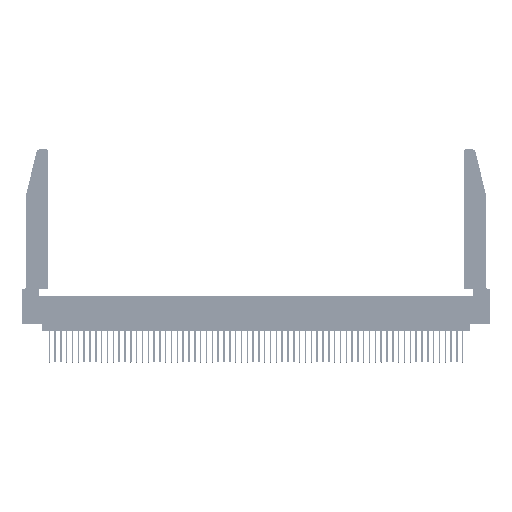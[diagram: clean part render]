
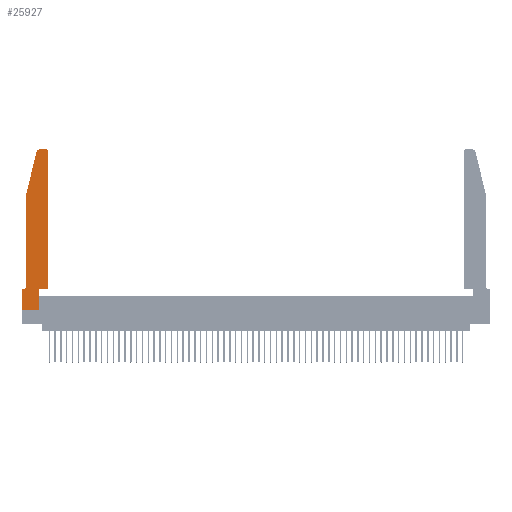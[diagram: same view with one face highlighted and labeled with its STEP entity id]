
A CAD part, top view. The second image highlights one B-rep face of the part: STEP entity #25927.
In plain terms, the highlighted planar face has unit normal (0, 0, 1).
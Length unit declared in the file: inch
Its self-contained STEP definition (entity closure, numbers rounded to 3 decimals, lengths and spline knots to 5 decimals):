
#822 = ORIENTED_EDGE ( 'NONE', *, *, #21798, .T. ) ;
#1445 = DIRECTION ( 'NONE',  ( -1., 0., 0. ) ) ;
#1590 = CARTESIAN_POINT ( 'NONE',  ( 0., 0., 0.37 ) ) ;
#1891 = CIRCLE ( 'NONE', #20197, 0.03 ) ;
#2078 = CARTESIAN_POINT ( 'NONE',  ( 0.4505, 0.35, 0.37 ) ) ;
#2247 = CARTESIAN_POINT ( 'NONE',  ( 0.0755, 2., 0.37 ) ) ;
#2632 = CARTESIAN_POINT ( 'NONE',  ( 0., 0., 0.37 ) ) ;
#2741 = ORIENTED_EDGE ( 'NONE', *, *, #57275, .T. ) ;
#3510 = ORIENTED_EDGE ( 'NONE', *, *, #42139, .T. ) ;
#3953 = VECTOR ( 'NONE', #46922, 39.37008 ) ;
#4458 = CARTESIAN_POINT ( 'NONE',  ( 0., 0.35, 0.37 ) ) ;
#5909 = EDGE_CURVE ( 'NONE', #23556, #12923, #20732, .T. ) ;
#6762 = LINE ( 'NONE', #46557, #3953 ) ;
#7547 = DIRECTION ( 'NONE',  ( -1., 0., 0. ) ) ;
#9109 = DIRECTION ( 'NONE',  ( 1., 0., 0. ) ) ;
#9307 = ORIENTED_EDGE ( 'NONE', *, *, #5909, .T. ) ;
#10715 = CARTESIAN_POINT ( 'NONE',  ( 0.2865, 0.35, 0.37 ) ) ;
#11379 = VERTEX_POINT ( 'NONE', #55346 ) ;
#11673 = LINE ( 'NONE', #27913, #43465 ) ;
#12029 = DIRECTION ( 'NONE',  ( 0., 0., 1. ) ) ;
#12777 = DIRECTION ( 'NONE',  ( 0., 0., 1. ) ) ;
#12923 = VERTEX_POINT ( 'NONE', #25942 ) ;
#13028 = CARTESIAN_POINT ( 'NONE',  ( 0.2865, 0., 0.37 ) ) ;
#13414 = VECTOR ( 'NONE', #33228, 39.37008 ) ;
#14267 = DIRECTION ( 'NONE',  ( 0., 1., 0. ) ) ;
#14324 = CARTESIAN_POINT ( 'NONE',  ( 0.25487, 2.72718, 0.37 ) ) ;
#14420 = VERTEX_POINT ( 'NONE', #1590 ) ;
#14425 = EDGE_LOOP ( 'NONE', ( #822, #54853, #9307, #50742, #24984, #39647, #30287, #35115, #42161, #19345, #3510, #2741 ) ) ;
#14500 = DIRECTION ( 'NONE',  ( 0., 0., 1. ) ) ;
#14911 = DIRECTION ( 'NONE',  ( 0., 1., 0. ) ) ;
#15782 = EDGE_CURVE ( 'NONE', #14420, #19353, #6762, .T. ) ;
#17158 = DIRECTION ( 'NONE',  ( -1., 0., 0. ) ) ;
#17532 = VERTEX_POINT ( 'NONE', #21543 ) ;
#18072 = VERTEX_POINT ( 'NONE', #38131 ) ;
#19186 = CARTESIAN_POINT ( 'NONE',  ( 0., 0.35, 0.37 ) ) ;
#19345 = ORIENTED_EDGE ( 'NONE', *, *, #22884, .T. ) ;
#19353 = VERTEX_POINT ( 'NONE', #13028 ) ;
#19830 = VECTOR ( 'NONE', #27950, 39.37008 ) ;
#20197 = AXIS2_PLACEMENT_3D ( 'NONE', #36756, #14500, #32133 ) ;
#20732 = LINE ( 'NONE', #27797, #24220 ) ;
#21417 = CARTESIAN_POINT ( 'NONE',  ( 0.0055, 0.42, 0.37 ) ) ;
#21543 = CARTESIAN_POINT ( 'NONE',  ( 0.284, 2.75, 0.37 ) ) ;
#21798 = EDGE_CURVE ( 'NONE', #43163, #17532, #23360, .T. ) ;
#22601 = VERTEX_POINT ( 'NONE', #25340 ) ;
#22884 = EDGE_CURVE ( 'NONE', #22601, #29561, #29512, .T. ) ;
#23360 = LINE ( 'NONE', #51400, #46912 ) ;
#23556 = VERTEX_POINT ( 'NONE', #14324 ) ;
#23658 = CARTESIAN_POINT ( 'NONE',  ( 0.4505, 0.35, 0.37 ) ) ;
#23695 = CARTESIAN_POINT ( 'NONE',  ( 0.0755, 0.35, 0.37 ) ) ;
#24220 = VECTOR ( 'NONE', #50194, 39.37008 ) ;
#24984 = ORIENTED_EDGE ( 'NONE', *, *, #41138, .T. ) ;
#25340 = CARTESIAN_POINT ( 'NONE',  ( 0.2865, 0.35, 0.37 ) ) ;
#25927 = ADVANCED_FACE ( 'NONE', ( #55930 ), #52606, .T. ) ;
#25942 = CARTESIAN_POINT ( 'NONE',  ( 0.0755, 2., 0.37 ) ) ;
#26031 = AXIS2_PLACEMENT_3D ( 'NONE', #21417, #29750, #17158 ) ;
#27797 = CARTESIAN_POINT ( 'NONE',  ( 0.0755, 2., 0.37 ) ) ;
#27913 = CARTESIAN_POINT ( 'NONE',  ( 0.4505, 0.35, 0.37 ) ) ;
#27950 = DIRECTION ( 'NONE',  ( 1., 0., 0. ) ) ;
#27963 = LINE ( 'NONE', #2632, #13414 ) ;
#28987 = VERTEX_POINT ( 'NONE', #19186 ) ;
#29512 = LINE ( 'NONE', #23658, #19830 ) ;
#29561 = VERTEX_POINT ( 'NONE', #2078 ) ;
#29750 = DIRECTION ( 'NONE',  ( 0., 0., -1. ) ) ;
#30287 = ORIENTED_EDGE ( 'NONE', *, *, #53662, .T. ) ;
#31819 = VECTOR ( 'NONE', #1445, 39.37008 ) ;
#32071 = CARTESIAN_POINT ( 'NONE',  ( 0.4205, 2.75, 0.37 ) ) ;
#32133 = DIRECTION ( 'NONE',  ( 1., 0., 0. ) ) ;
#33228 = DIRECTION ( 'NONE',  ( 0., -1., 0. ) ) ;
#34633 = VECTOR ( 'NONE', #14267, 39.37008 ) ;
#35115 = ORIENTED_EDGE ( 'NONE', *, *, #15782, .T. ) ;
#35244 = CIRCLE ( 'NONE', #39544, 0.03 ) ;
#35970 = LINE ( 'NONE', #23695, #31819 ) ;
#36756 = CARTESIAN_POINT ( 'NONE',  ( 0.284, 2.72, 0.37 ) ) ;
#37843 = AXIS2_PLACEMENT_3D ( 'NONE', #4458, #12777, #9109 ) ;
#38131 = CARTESIAN_POINT ( 'NONE',  ( 0.0055, 0.35, 0.37 ) ) ;
#38988 = EDGE_CURVE ( 'NONE', #12923, #54003, #41715, .T. ) ;
#39544 = AXIS2_PLACEMENT_3D ( 'NONE', #51073, #12029, #46650 ) ;
#39647 = ORIENTED_EDGE ( 'NONE', *, *, #56484, .T. ) ;
#41138 = EDGE_CURVE ( 'NONE', #54003, #18072, #47741, .T. ) ;
#41715 = LINE ( 'NONE', #2247, #55591 ) ;
#42139 = EDGE_CURVE ( 'NONE', #29561, #11379, #11673, .T. ) ;
#42161 = ORIENTED_EDGE ( 'NONE', *, *, #56404, .T. ) ;
#42704 = EDGE_CURVE ( 'NONE', #17532, #23556, #1891, .T. ) ;
#43163 = VERTEX_POINT ( 'NONE', #32071 ) ;
#43432 = CARTESIAN_POINT ( 'NONE',  ( 0.0755, 0.42, 0.37 ) ) ;
#43465 = VECTOR ( 'NONE', #14911, 39.37008 ) ;
#46394 = LINE ( 'NONE', #10715, #34633 ) ;
#46557 = CARTESIAN_POINT ( 'NONE',  ( 0., 0., 0.37 ) ) ;
#46650 = DIRECTION ( 'NONE',  ( 1., 0., 0. ) ) ;
#46912 = VECTOR ( 'NONE', #7547, 39.37008 ) ;
#46922 = DIRECTION ( 'NONE',  ( 1., 0., 0. ) ) ;
#47741 = CIRCLE ( 'NONE', #26031, 0.07 ) ;
#50194 = DIRECTION ( 'NONE',  ( -0.239, -0.971, 0. ) ) ;
#50742 = ORIENTED_EDGE ( 'NONE', *, *, #38988, .T. ) ;
#51073 = CARTESIAN_POINT ( 'NONE',  ( 0.4205, 2.72, 0.37 ) ) ;
#51400 = CARTESIAN_POINT ( 'NONE',  ( 0.2605, 2.75, 0.37 ) ) ;
#52606 = PLANE ( 'NONE',  #37843 ) ;
#53662 = EDGE_CURVE ( 'NONE', #28987, #14420, #27963, .T. ) ;
#54003 = VERTEX_POINT ( 'NONE', #43432 ) ;
#54853 = ORIENTED_EDGE ( 'NONE', *, *, #42704, .T. ) ;
#55346 = CARTESIAN_POINT ( 'NONE',  ( 0.4505, 2.72, 0.37 ) ) ;
#55591 = VECTOR ( 'NONE', #55658, 39.37008 ) ;
#55658 = DIRECTION ( 'NONE',  ( 0., -1., 0. ) ) ;
#55930 = FACE_OUTER_BOUND ( 'NONE', #14425, .T. ) ;
#56404 = EDGE_CURVE ( 'NONE', #19353, #22601, #46394, .T. ) ;
#56484 = EDGE_CURVE ( 'NONE', #18072, #28987, #35970, .T. ) ;
#57275 = EDGE_CURVE ( 'NONE', #11379, #43163, #35244, .T. ) ;
